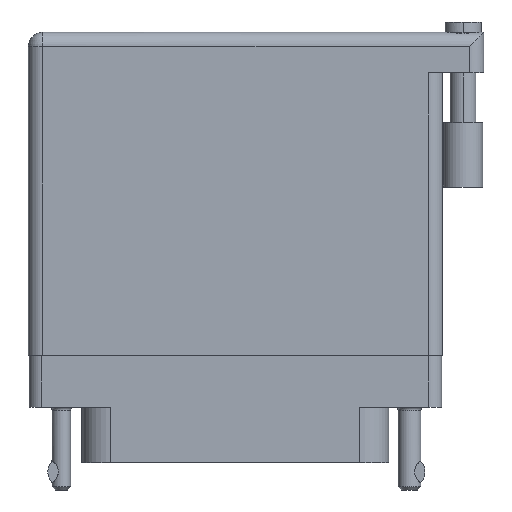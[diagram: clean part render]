
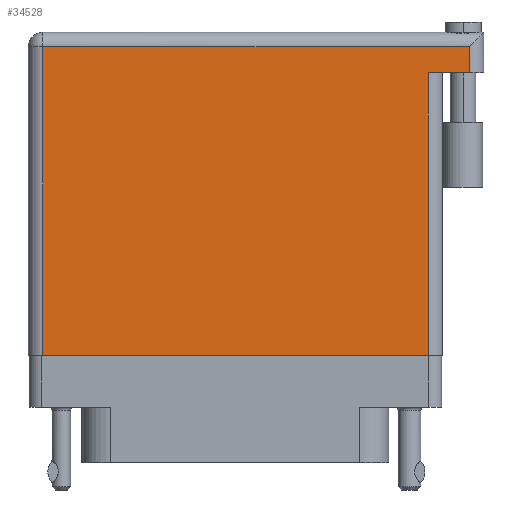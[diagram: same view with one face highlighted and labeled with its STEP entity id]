
A CAD part, front view. The second image highlights one B-rep face of the part: STEP entity #34528.
In plain terms, the highlighted face is planar.
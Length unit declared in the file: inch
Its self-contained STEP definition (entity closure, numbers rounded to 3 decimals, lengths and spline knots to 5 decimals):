
#4260 = DIRECTION ( 'NONE',  ( 1., 0., 0. ) ) ;
#4770 = VECTOR ( 'NONE', #37270, 39.37008 ) ;
#5977 = ORIENTED_EDGE ( 'NONE', *, *, #32290, .T. ) ;
#6075 = ORIENTED_EDGE ( 'NONE', *, *, #17730, .T. ) ;
#6729 = CARTESIAN_POINT ( 'NONE',  ( 1.134, 1.466, 0.4495 ) ) ;
#6864 = LINE ( 'NONE', #6729, #9206 ) ;
#7456 = DIRECTION ( 'NONE',  ( 0., -1., 0. ) ) ;
#8777 = VECTOR ( 'NONE', #7456, 39.37008 ) ;
#9206 = VECTOR ( 'NONE', #21455, 39.37008 ) ;
#9439 = ORIENTED_EDGE ( 'NONE', *, *, #32947, .T. ) ;
#10761 = CARTESIAN_POINT ( 'NONE',  ( -0.934, -0.1, 0.4495 ) ) ;
#13353 = EDGE_LOOP ( 'NONE', ( #5977, #20779, #41590, #9439, #13612, #6075 ) ) ;
#13612 = ORIENTED_EDGE ( 'NONE', *, *, #25013, .T. ) ;
#14554 = LINE ( 'NONE', #32992, #22255 ) ;
#16411 = LINE ( 'NONE', #23279, #46111 ) ;
#17730 = EDGE_CURVE ( 'NONE', #45788, #22666, #40802, .T. ) ;
#17772 = DIRECTION ( 'NONE',  ( -1., 0., 0. ) ) ;
#17981 = VERTEX_POINT ( 'NONE', #46398 ) ;
#19757 = VECTOR ( 'NONE', #17772, 39.37008 ) ;
#20505 = VERTEX_POINT ( 'NONE', #47678 ) ;
#20779 = ORIENTED_EDGE ( 'NONE', *, *, #21751, .T. ) ;
#21455 = DIRECTION ( 'NONE',  ( 0., 1., 0. ) ) ;
#21751 = EDGE_CURVE ( 'NONE', #20505, #28035, #14554, .T. ) ;
#22255 = VECTOR ( 'NONE', #36965, 39.37008 ) ;
#22399 = DIRECTION ( 'NONE',  ( 0., 0., -1. ) ) ;
#22666 = VERTEX_POINT ( 'NONE', #43419 ) ;
#23279 = CARTESIAN_POINT ( 'NONE',  ( -1.004, -0.1, 0.4495 ) ) ;
#25013 = EDGE_CURVE ( 'NONE', #40657, #45788, #48028, .T. ) ;
#25253 = CARTESIAN_POINT ( 'NONE',  ( -0.934, 1.396, 0.4495 ) ) ;
#25854 = PLANE ( 'NONE',  #25913 ) ;
#25913 = AXIS2_PLACEMENT_3D ( 'NONE', #37848, #22399, #37512 ) ;
#26675 = CARTESIAN_POINT ( 'NONE',  ( 1.134, 1.396, 0.4495 ) ) ;
#27414 = CARTESIAN_POINT ( 'NONE',  ( 0.934, 1.269, 0.4495 ) ) ;
#28035 = VERTEX_POINT ( 'NONE', #27414 ) ;
#32290 = EDGE_CURVE ( 'NONE', #22666, #20505, #16411, .T. ) ;
#32947 = EDGE_CURVE ( 'NONE', #17981, #40657, #6864, .T. ) ;
#32992 = CARTESIAN_POINT ( 'NONE',  ( 0.934, 1.269, 0.4495 ) ) ;
#34528 = ADVANCED_FACE ( 'NONE', ( #40526 ), #25854, .F. ) ;
#35783 = LINE ( 'NONE', #47758, #19757 ) ;
#36965 = DIRECTION ( 'NONE',  ( 0., 1., 0. ) ) ;
#37270 = DIRECTION ( 'NONE',  ( -1., 0., 0. ) ) ;
#37512 = DIRECTION ( 'NONE',  ( -1., 0., 0. ) ) ;
#37848 = CARTESIAN_POINT ( 'NONE',  ( -1.004, 1.466, 0.4495 ) ) ;
#40088 = CARTESIAN_POINT ( 'NONE',  ( -1.004, 1.396, 0.4495 ) ) ;
#40526 = FACE_OUTER_BOUND ( 'NONE', #13353, .T. ) ;
#40657 = VERTEX_POINT ( 'NONE', #26675 ) ;
#40802 = LINE ( 'NONE', #10761, #8777 ) ;
#40862 = EDGE_CURVE ( 'NONE', #17981, #28035, #35783, .T. ) ;
#41590 = ORIENTED_EDGE ( 'NONE', *, *, #40862, .F. ) ;
#43419 = CARTESIAN_POINT ( 'NONE',  ( -0.934, -0.1, 0.4495 ) ) ;
#45788 = VERTEX_POINT ( 'NONE', #25253 ) ;
#46111 = VECTOR ( 'NONE', #4260, 39.37008 ) ;
#46398 = CARTESIAN_POINT ( 'NONE',  ( 1.134, 1.269, 0.4495 ) ) ;
#47678 = CARTESIAN_POINT ( 'NONE',  ( 0.934, -0.1, 0.4495 ) ) ;
#47758 = CARTESIAN_POINT ( 'NONE',  ( 1.204, 1.269, 0.4495 ) ) ;
#48028 = LINE ( 'NONE', #40088, #4770 ) ;
